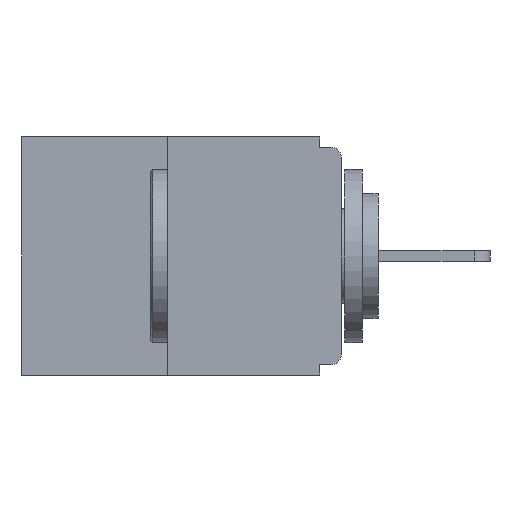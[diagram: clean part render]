
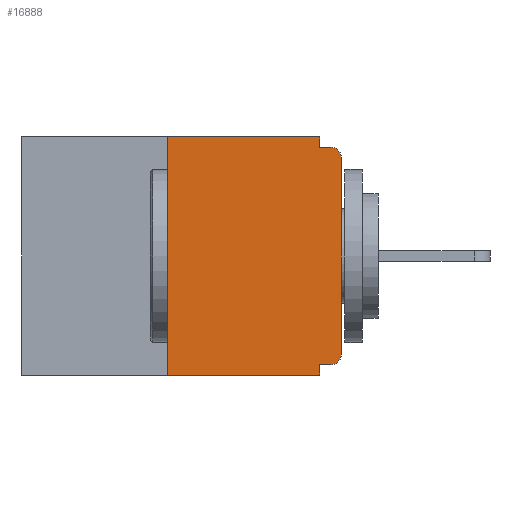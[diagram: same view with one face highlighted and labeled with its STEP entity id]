
A CAD part, left-side view. The second image highlights one B-rep face of the part: STEP entity #16888.
In plain terms, the highlighted planar face has unit normal (-1, 0, 0).
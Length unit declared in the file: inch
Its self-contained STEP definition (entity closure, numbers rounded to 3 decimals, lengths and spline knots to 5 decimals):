
#617 = CARTESIAN_POINT ( 'NONE',  ( 0., 0., -0.015 ) ) ;
#861 = CARTESIAN_POINT ( 'NONE',  ( 0., 0.031, -0.328 ) ) ;
#868 = CARTESIAN_POINT ( 'NONE',  ( 0., 0.015, -0.328 ) ) ;
#1093 = LINE ( 'NONE', #4630, #1569 ) ;
#1104 = CARTESIAN_POINT ( 'NONE',  ( 0., 0.015, -0.313 ) ) ;
#1167 = LINE ( 'NONE', #10496, #16044 ) ;
#1186 = EDGE_LOOP ( 'NONE', ( #9452, #14696, #11276, #1570, #5912, #14920, #15345, #9921, #10377, #4558 ) ) ;
#1569 = VECTOR ( 'NONE', #14723, 39.37008 ) ;
#1570 = ORIENTED_EDGE ( 'NONE', *, *, #6799, .F. ) ;
#1711 = DIRECTION ( 'NONE',  ( 0., 0., 1. ) ) ;
#1932 = VERTEX_POINT ( 'NONE', #13334 ) ;
#2195 = VECTOR ( 'NONE', #6513, 39.37008 ) ;
#2572 = DIRECTION ( 'NONE',  ( 0., 0., -1. ) ) ;
#2655 = VERTEX_POINT ( 'NONE', #13480 ) ;
#2783 = CARTESIAN_POINT ( 'NONE',  ( 0., 0., 0. ) ) ;
#2869 = VECTOR ( 'NONE', #3851, 39.37008 ) ;
#2990 = VERTEX_POINT ( 'NONE', #15682 ) ;
#3173 = AXIS2_PLACEMENT_3D ( 'NONE', #1104, #11219, #2572 ) ;
#3349 = VECTOR ( 'NONE', #16043, 39.37008 ) ;
#3646 = CIRCLE ( 'NONE', #3173, 0.015 ) ;
#3681 = EDGE_CURVE ( 'NONE', #8046, #2655, #6103, .T. ) ;
#3851 = DIRECTION ( 'NONE',  ( 0., -1., 0. ) ) ;
#3948 = CARTESIAN_POINT ( 'NONE',  ( 0., 0.46, 0. ) ) ;
#4370 = EDGE_CURVE ( 'NONE', #2990, #1932, #13967, .T. ) ;
#4388 = VERTEX_POINT ( 'NONE', #861 ) ;
#4389 = DIRECTION ( 'NONE',  ( 0., 0., -1. ) ) ;
#4403 = DIRECTION ( 'NONE',  ( -1., 0., 0. ) ) ;
#4454 = CARTESIAN_POINT ( 'NONE',  ( 0., 0.015, -0.03 ) ) ;
#4558 = ORIENTED_EDGE ( 'NONE', *, *, #9139, .F. ) ;
#4630 = CARTESIAN_POINT ( 'NONE',  ( 0., 0.46, 0. ) ) ;
#5414 = DIRECTION ( 'NONE',  ( 1., 0., 0. ) ) ;
#5912 = ORIENTED_EDGE ( 'NONE', *, *, #6359, .F. ) ;
#6103 = LINE ( 'NONE', #7767, #2195 ) ;
#6359 = EDGE_CURVE ( 'NONE', #13814, #4388, #14888, .T. ) ;
#6500 = VECTOR ( 'NONE', #1711, 39.37008 ) ;
#6513 = DIRECTION ( 'NONE',  ( 0., -1., 0. ) ) ;
#6696 = EDGE_CURVE ( 'NONE', #8046, #17220, #9415, .T. ) ;
#6799 = EDGE_CURVE ( 'NONE', #4388, #2655, #7194, .T. ) ;
#6946 = LINE ( 'NONE', #2783, #6500 ) ;
#7167 = AXIS2_PLACEMENT_3D ( 'NONE', #3948, #5414, #15459 ) ;
#7194 = LINE ( 'NONE', #16057, #3349 ) ;
#7351 = EDGE_CURVE ( 'NONE', #16010, #1932, #12135, .T. ) ;
#7486 = EDGE_CURVE ( 'NONE', #12462, #16010, #6946, .T. ) ;
#7767 = CARTESIAN_POINT ( 'NONE',  ( 0., 0.46, -0.343 ) ) ;
#8046 = VERTEX_POINT ( 'NONE', #16446 ) ;
#8998 = VECTOR ( 'NONE', #15531, 39.37008 ) ;
#9139 = EDGE_CURVE ( 'NONE', #14517, #2990, #1167, .T. ) ;
#9415 = LINE ( 'NONE', #18107, #14200 ) ;
#9452 = ORIENTED_EDGE ( 'NONE', *, *, #12148, .F. ) ;
#9921 = ORIENTED_EDGE ( 'NONE', *, *, #7351, .T. ) ;
#10019 = CARTESIAN_POINT ( 'NONE',  ( 0., 0.031, 0. ) ) ;
#10377 = ORIENTED_EDGE ( 'NONE', *, *, #4370, .F. ) ;
#10496 = CARTESIAN_POINT ( 'NONE',  ( 0., 0.031, 0. ) ) ;
#10654 = CARTESIAN_POINT ( 'NONE',  ( 0., 0., -0.03 ) ) ;
#11219 = DIRECTION ( 'NONE',  ( -1., 0., 0. ) ) ;
#11276 = ORIENTED_EDGE ( 'NONE', *, *, #3681, .T. ) ;
#12081 = CARTESIAN_POINT ( 'NONE',  ( 0., 0.25, 0. ) ) ;
#12135 = CIRCLE ( 'NONE', #12280, 0.015 ) ;
#12148 = EDGE_CURVE ( 'NONE', #17220, #14517, #1093, .T. ) ;
#12280 = AXIS2_PLACEMENT_3D ( 'NONE', #4454, #4403, #4389 ) ;
#12462 = VERTEX_POINT ( 'NONE', #12692 ) ;
#12692 = CARTESIAN_POINT ( 'NONE',  ( 0., 0., -0.313 ) ) ;
#13334 = CARTESIAN_POINT ( 'NONE',  ( 0., 0.015, -0.015 ) ) ;
#13480 = CARTESIAN_POINT ( 'NONE',  ( 0., 0.031, -0.343 ) ) ;
#13814 = VERTEX_POINT ( 'NONE', #868 ) ;
#13967 = LINE ( 'NONE', #617, #2869 ) ;
#14200 = VECTOR ( 'NONE', #18055, 39.37008 ) ;
#14517 = VERTEX_POINT ( 'NONE', #10019 ) ;
#14696 = ORIENTED_EDGE ( 'NONE', *, *, #6696, .F. ) ;
#14723 = DIRECTION ( 'NONE',  ( 0., -1., 0. ) ) ;
#14888 = LINE ( 'NONE', #15804, #8998 ) ;
#14898 = DIRECTION ( 'NONE',  ( 0., 0., -1. ) ) ;
#14920 = ORIENTED_EDGE ( 'NONE', *, *, #17457, .T. ) ;
#15345 = ORIENTED_EDGE ( 'NONE', *, *, #7486, .T. ) ;
#15459 = DIRECTION ( 'NONE',  ( 0., 0., -1. ) ) ;
#15531 = DIRECTION ( 'NONE',  ( 0., 1., 0. ) ) ;
#15682 = CARTESIAN_POINT ( 'NONE',  ( 0., 0.031, -0.015 ) ) ;
#15804 = CARTESIAN_POINT ( 'NONE',  ( 0., 0., -0.328 ) ) ;
#16010 = VERTEX_POINT ( 'NONE', #10654 ) ;
#16043 = DIRECTION ( 'NONE',  ( 0., 0., -1. ) ) ;
#16044 = VECTOR ( 'NONE', #14898, 39.37008 ) ;
#16057 = CARTESIAN_POINT ( 'NONE',  ( 0., 0.031, -0.343 ) ) ;
#16446 = CARTESIAN_POINT ( 'NONE',  ( 0., 0.25, -0.343 ) ) ;
#16888 = ADVANCED_FACE ( 'NONE', ( #17884 ), #18095, .F. ) ;
#17220 = VERTEX_POINT ( 'NONE', #12081 ) ;
#17457 = EDGE_CURVE ( 'NONE', #13814, #12462, #3646, .T. ) ;
#17884 = FACE_OUTER_BOUND ( 'NONE', #1186, .T. ) ;
#18055 = DIRECTION ( 'NONE',  ( 0., 0., 1. ) ) ;
#18095 = PLANE ( 'NONE',  #7167 ) ;
#18107 = CARTESIAN_POINT ( 'NONE',  ( 0., 0.25, 0. ) ) ;
